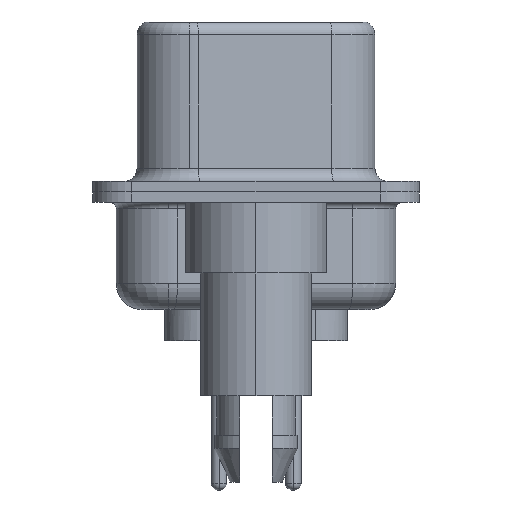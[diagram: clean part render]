
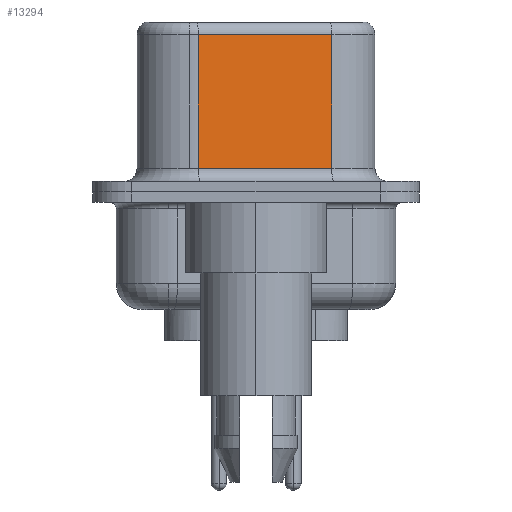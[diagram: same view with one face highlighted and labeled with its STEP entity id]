
A CAD part, left-side view. The second image highlights one B-rep face of the part: STEP entity #13294.
In plain terms, the highlighted planar face has unit normal (-0.985, -0.174, 0).
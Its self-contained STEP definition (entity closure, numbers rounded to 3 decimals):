
#57 = DIRECTION ( 'NONE',  ( 0., 0., -1. ) ) ;
#183 = CARTESIAN_POINT ( 'NONE',  ( 3.655, 2.203, 0.9 ) ) ;
#297 = DIRECTION ( 'NONE',  ( 0., 0., -1. ) ) ;
#316 = CARTESIAN_POINT ( 'NONE',  ( 4.555, -2.897, 6.52 ) ) ;
#4201 = DIRECTION ( 'NONE',  ( 0.985, 0.174, 0. ) ) ;
#4378 = ORIENTED_EDGE ( 'NONE', *, *, #5132, .T. ) ;
#4451 = DIRECTION ( 'NONE',  ( -0.174, 0.985, 0. ) ) ;
#5132 = EDGE_CURVE ( 'NONE', #17775, #15181, #16625, .T. ) ;
#5729 = FACE_OUTER_BOUND ( 'NONE', #13418, .T. ) ;
#6200 = DIRECTION ( 'NONE',  ( -0.174, 0.985, 0. ) ) ;
#6750 = VERTEX_POINT ( 'NONE', #13544 ) ;
#6812 = DIRECTION ( 'NONE',  ( 0.174, -0.985, 0. ) ) ;
#6901 = LINE ( 'NONE', #7075, #7040 ) ;
#7040 = VECTOR ( 'NONE', #6812, 1000. ) ;
#7075 = CARTESIAN_POINT ( 'NONE',  ( 4.555, -2.897, 0.9 ) ) ;
#7723 = ORIENTED_EDGE ( 'NONE', *, *, #12093, .T. ) ;
#8182 = VECTOR ( 'NONE', #57, 1000. ) ;
#9065 = CARTESIAN_POINT ( 'NONE',  ( 4.555, -2.897, 6.02 ) ) ;
#9930 = CARTESIAN_POINT ( 'NONE',  ( 3.655, 2.203, 6.52 ) ) ;
#10118 = ORIENTED_EDGE ( 'NONE', *, *, #13346, .T. ) ;
#10367 = VERTEX_POINT ( 'NONE', #12237 ) ;
#12093 = EDGE_CURVE ( 'NONE', #10367, #17775, #14417, .T. ) ;
#12237 = CARTESIAN_POINT ( 'NONE',  ( 4.555, -2.897, 6.02 ) ) ;
#12927 = ORIENTED_EDGE ( 'NONE', *, *, #13252, .F. ) ;
#13252 = EDGE_CURVE ( 'NONE', #10367, #6750, #16467, .T. ) ;
#13294 = ADVANCED_FACE ( 'NONE', ( #5729 ), #13947, .F. ) ;
#13346 = EDGE_CURVE ( 'NONE', #15181, #6750, #6901, .T. ) ;
#13418 = EDGE_LOOP ( 'NONE', ( #12927, #7723, #4378, #10118 ) ) ;
#13544 = CARTESIAN_POINT ( 'NONE',  ( 4.555, -2.897, 0.9 ) ) ;
#13657 = CARTESIAN_POINT ( 'NONE',  ( 3.655, 2.203, 6.02 ) ) ;
#13681 = CARTESIAN_POINT ( 'NONE',  ( 4.555, -2.897, 6.52 ) ) ;
#13936 = VECTOR ( 'NONE', #6200, 1000. ) ;
#13947 = PLANE ( 'NONE',  #15106 ) ;
#14417 = LINE ( 'NONE', #9065, #13936 ) ;
#15106 = AXIS2_PLACEMENT_3D ( 'NONE', #316, #4201, #4451 ) ;
#15181 = VERTEX_POINT ( 'NONE', #183 ) ;
#16467 = LINE ( 'NONE', #13681, #8182 ) ;
#16625 = LINE ( 'NONE', #9930, #16975 ) ;
#16975 = VECTOR ( 'NONE', #297, 1000. ) ;
#17775 = VERTEX_POINT ( 'NONE', #13657 ) ;
